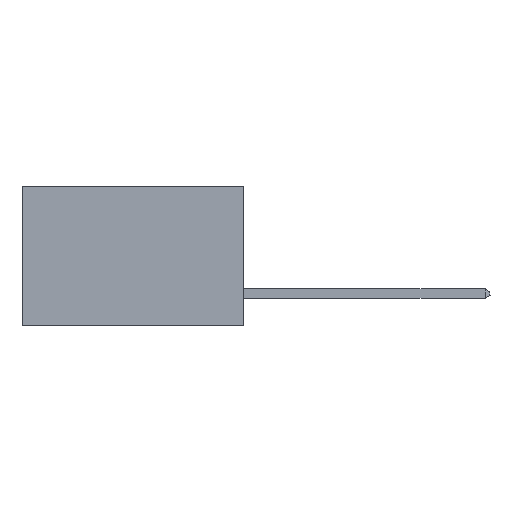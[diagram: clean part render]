
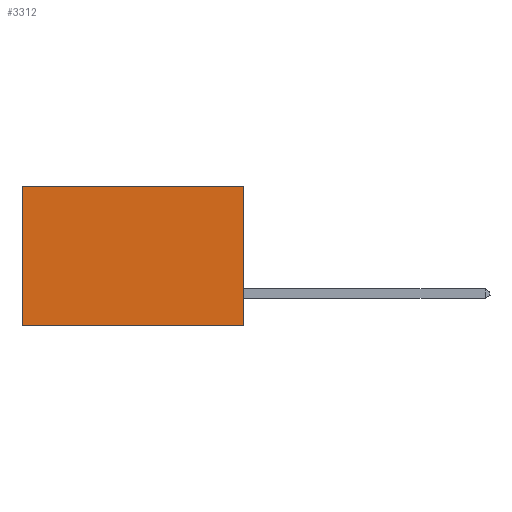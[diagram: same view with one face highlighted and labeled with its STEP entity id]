
A CAD part, left-side view. The second image highlights one B-rep face of the part: STEP entity #3312.
In plain terms, the highlighted planar face has unit normal (-1, 0, 0).
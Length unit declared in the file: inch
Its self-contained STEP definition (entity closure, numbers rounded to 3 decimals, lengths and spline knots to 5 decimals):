
#326 = VERTEX_POINT ( 'NONE', #7995 ) ;
#905 = EDGE_CURVE ( 'NONE', #10354, #11166, #7032, .T. ) ;
#1098 = EDGE_LOOP ( 'NONE', ( #10569, #8792, #8767, #8742 ) ) ;
#1120 = EDGE_CURVE ( 'NONE', #10354, #326, #3189, .T. ) ;
#1845 = CARTESIAN_POINT ( 'NONE',  ( 0.277, 0.59, 0. ) ) ;
#2914 = PLANE ( 'NONE',  #5250 ) ;
#2918 = DIRECTION ( 'NONE',  ( 1., 0., 0. ) ) ;
#2996 = LINE ( 'NONE', #4287, #9219 ) ;
#3189 = LINE ( 'NONE', #3627, #4900 ) ;
#3312 = ADVANCED_FACE ( 'NONE', ( #5090 ), #2914, .F. ) ;
#3542 = EDGE_CURVE ( 'NONE', #326, #6659, #2996, .T. ) ;
#3619 = EDGE_CURVE ( 'NONE', #11166, #6659, #6401, .T. ) ;
#3627 = CARTESIAN_POINT ( 'NONE',  ( 0.277, 0., -0.37 ) ) ;
#4287 = CARTESIAN_POINT ( 'NONE',  ( 0.277, 0., -0.37 ) ) ;
#4431 = CARTESIAN_POINT ( 'NONE',  ( 0.277, 0., 0. ) ) ;
#4462 = DIRECTION ( 'NONE',  ( 0., 0., -1. ) ) ;
#4769 = VECTOR ( 'NONE', #6443, 39.37008 ) ;
#4900 = VECTOR ( 'NONE', #4462, 39.37008 ) ;
#5090 = FACE_OUTER_BOUND ( 'NONE', #1098, .T. ) ;
#5250 = AXIS2_PLACEMENT_3D ( 'NONE', #9787, #2918, #9022 ) ;
#5678 = DIRECTION ( 'NONE',  ( 0., 1., 0. ) ) ;
#5762 = CARTESIAN_POINT ( 'NONE',  ( 0.277, 0.59, -0.37 ) ) ;
#6401 = LINE ( 'NONE', #5762, #8430 ) ;
#6443 = DIRECTION ( 'NONE',  ( 0., 1., 0. ) ) ;
#6520 = CARTESIAN_POINT ( 'NONE',  ( 0.277, 0., 0. ) ) ;
#6659 = VERTEX_POINT ( 'NONE', #9162 ) ;
#7032 = LINE ( 'NONE', #4431, #4769 ) ;
#7995 = CARTESIAN_POINT ( 'NONE',  ( 0.277, 0., -0.37 ) ) ;
#8430 = VECTOR ( 'NONE', #9108, 39.37008 ) ;
#8742 = ORIENTED_EDGE ( 'NONE', *, *, #905, .T. ) ;
#8767 = ORIENTED_EDGE ( 'NONE', *, *, #1120, .F. ) ;
#8792 = ORIENTED_EDGE ( 'NONE', *, *, #3542, .F. ) ;
#9022 = DIRECTION ( 'NONE',  ( 0., 0., -1. ) ) ;
#9108 = DIRECTION ( 'NONE',  ( 0., 0., -1. ) ) ;
#9162 = CARTESIAN_POINT ( 'NONE',  ( 0.277, 0.59, -0.37 ) ) ;
#9219 = VECTOR ( 'NONE', #5678, 39.37008 ) ;
#9787 = CARTESIAN_POINT ( 'NONE',  ( 0.277, 0., -0.37 ) ) ;
#10354 = VERTEX_POINT ( 'NONE', #6520 ) ;
#10569 = ORIENTED_EDGE ( 'NONE', *, *, #3619, .T. ) ;
#11166 = VERTEX_POINT ( 'NONE', #1845 ) ;
